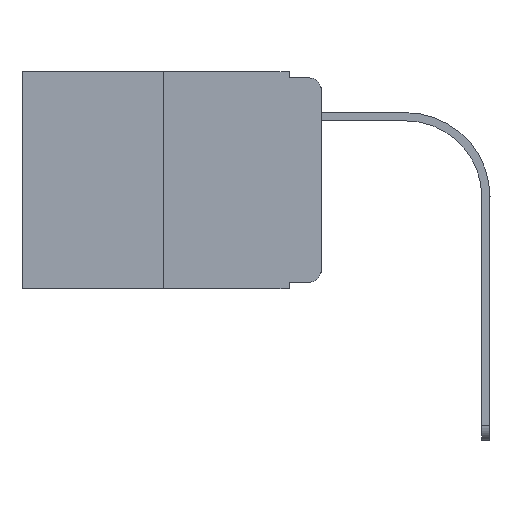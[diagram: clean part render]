
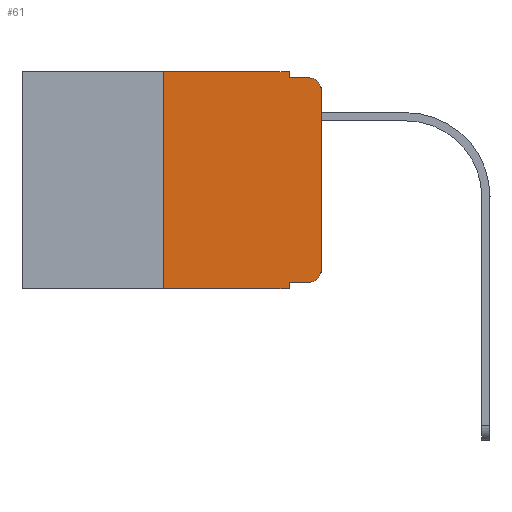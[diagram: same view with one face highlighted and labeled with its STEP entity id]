
A CAD part, left-side view. The second image highlights one B-rep face of the part: STEP entity #61.
In plain terms, the highlighted planar face has unit normal (-1, 0, 0).
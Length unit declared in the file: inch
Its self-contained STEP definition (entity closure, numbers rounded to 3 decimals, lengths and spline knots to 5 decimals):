
#28 = EDGE_CURVE ( 'NONE', #7115, #13252, #396, .T. ) ;
#61 = ADVANCED_FACE ( 'NONE', ( #12761 ), #3958, .F. ) ;
#110 = ORIENTED_EDGE ( 'NONE', *, *, #10447, .T. ) ;
#242 = VECTOR ( 'NONE', #22299, 39.37008 ) ;
#321 = CARTESIAN_POINT ( 'NONE',  ( 0., 0., -0.313 ) ) ;
#396 = LINE ( 'NONE', #7620, #4581 ) ;
#743 = CARTESIAN_POINT ( 'NONE',  ( 0., 0.02, -0.333 ) ) ;
#991 = VERTEX_POINT ( 'NONE', #19166 ) ;
#1076 = CARTESIAN_POINT ( 'NONE',  ( 0., 0.051, -0.333 ) ) ;
#1515 = DIRECTION ( 'NONE',  ( 0., -1., 0. ) ) ;
#1813 = EDGE_CURVE ( 'NONE', #22395, #3302, #22388, .T. ) ;
#1983 = LINE ( 'NONE', #7271, #15126 ) ;
#2420 = ORIENTED_EDGE ( 'NONE', *, *, #20080, .T. ) ;
#2516 = CARTESIAN_POINT ( 'NONE',  ( 0., 0.051, -0.333 ) ) ;
#2645 = CARTESIAN_POINT ( 'NONE',  ( 0., 0.051, 0. ) ) ;
#3045 = VERTEX_POINT ( 'NONE', #3527 ) ;
#3098 = EDGE_CURVE ( 'NONE', #14283, #3302, #21057, .T. ) ;
#3302 = VERTEX_POINT ( 'NONE', #5292 ) ;
#3527 = CARTESIAN_POINT ( 'NONE',  ( 0., 0.25, 0. ) ) ;
#3554 = CARTESIAN_POINT ( 'NONE',  ( 0., 0.25, 0. ) ) ;
#3932 = CIRCLE ( 'NONE', #8331, 0.02 ) ;
#3958 = PLANE ( 'NONE',  #19962 ) ;
#4429 = CARTESIAN_POINT ( 'NONE',  ( 0., 0.02, -0.03 ) ) ;
#4581 = VECTOR ( 'NONE', #19763, 39.37008 ) ;
#4913 = ORIENTED_EDGE ( 'NONE', *, *, #14765, .T. ) ;
#4995 = DIRECTION ( 'NONE',  ( 0., -1., 0. ) ) ;
#5292 = CARTESIAN_POINT ( 'NONE',  ( 0., 0.051, -0.343 ) ) ;
#5351 = CARTESIAN_POINT ( 'NONE',  ( 0., 0.051, 0. ) ) ;
#6211 = ORIENTED_EDGE ( 'NONE', *, *, #28, .F. ) ;
#6414 = AXIS2_PLACEMENT_3D ( 'NONE', #4429, #21852, #18425 ) ;
#6706 = CARTESIAN_POINT ( 'NONE',  ( 0., 0.473, -0.343 ) ) ;
#7115 = VERTEX_POINT ( 'NONE', #2645 ) ;
#7271 = CARTESIAN_POINT ( 'NONE',  ( 0., 0.473, 0. ) ) ;
#7287 = VERTEX_POINT ( 'NONE', #321 ) ;
#7439 = ORIENTED_EDGE ( 'NONE', *, *, #11410, .F. ) ;
#7620 = CARTESIAN_POINT ( 'NONE',  ( 0., 0.051, 0. ) ) ;
#7662 = ORIENTED_EDGE ( 'NONE', *, *, #3098, .F. ) ;
#8331 = AXIS2_PLACEMENT_3D ( 'NONE', #9095, #17698, #16332 ) ;
#8520 = CARTESIAN_POINT ( 'NONE',  ( 0., 0., 0. ) ) ;
#8583 = VERTEX_POINT ( 'NONE', #743 ) ;
#9095 = CARTESIAN_POINT ( 'NONE',  ( 0., 0.02, -0.313 ) ) ;
#9356 = DIRECTION ( 'NONE',  ( 0., 0., 1. ) ) ;
#9366 = VECTOR ( 'NONE', #4995, 39.37008 ) ;
#9940 = CARTESIAN_POINT ( 'NONE',  ( 0., 0.051, -0.01 ) ) ;
#10380 = CARTESIAN_POINT ( 'NONE',  ( 0., 0.051, -0.01 ) ) ;
#10447 = EDGE_CURVE ( 'NONE', #14283, #8583, #17235, .T. ) ;
#10637 = ORIENTED_EDGE ( 'NONE', *, *, #16602, .T. ) ;
#10939 = CARTESIAN_POINT ( 'NONE',  ( 0., 0.473, 0. ) ) ;
#11410 = EDGE_CURVE ( 'NONE', #3045, #7115, #1983, .T. ) ;
#11481 = CARTESIAN_POINT ( 'NONE',  ( 0., 0.25, -0.343 ) ) ;
#12341 = DIRECTION ( 'NONE',  ( 0., 0., -1. ) ) ;
#12761 = FACE_OUTER_BOUND ( 'NONE', #18529, .T. ) ;
#12916 = EDGE_CURVE ( 'NONE', #22395, #3045, #19781, .T. ) ;
#13252 = VERTEX_POINT ( 'NONE', #10380 ) ;
#13697 = VECTOR ( 'NONE', #9356, 39.37008 ) ;
#14283 = VERTEX_POINT ( 'NONE', #2516 ) ;
#14428 = VECTOR ( 'NONE', #21222, 39.37008 ) ;
#14724 = DIRECTION ( 'NONE',  ( 0., 0., -1. ) ) ;
#14765 = EDGE_CURVE ( 'NONE', #15584, #991, #16297, .T. ) ;
#15126 = VECTOR ( 'NONE', #16201, 39.37008 ) ;
#15353 = LINE ( 'NONE', #9940, #242 ) ;
#15584 = VERTEX_POINT ( 'NONE', #20282 ) ;
#16075 = EDGE_CURVE ( 'NONE', #13252, #991, #15353, .T. ) ;
#16201 = DIRECTION ( 'NONE',  ( 0., -1., 0. ) ) ;
#16297 = CIRCLE ( 'NONE', #6414, 0.02 ) ;
#16332 = DIRECTION ( 'NONE',  ( 0., 0., -1. ) ) ;
#16602 = EDGE_CURVE ( 'NONE', #8583, #7287, #3932, .T. ) ;
#17235 = LINE ( 'NONE', #1076, #18387 ) ;
#17516 = VECTOR ( 'NONE', #12341, 39.37008 ) ;
#17698 = DIRECTION ( 'NONE',  ( -1., 0., 0. ) ) ;
#17948 = DIRECTION ( 'NONE',  ( 1., 0., 0. ) ) ;
#18387 = VECTOR ( 'NONE', #1515, 39.37008 ) ;
#18425 = DIRECTION ( 'NONE',  ( 0., 0., -1. ) ) ;
#18529 = EDGE_LOOP ( 'NONE', ( #2420, #4913, #20936, #6211, #7439, #20776, #21105, #7662, #110, #10637 ) ) ;
#19166 = CARTESIAN_POINT ( 'NONE',  ( 0., 0.02, -0.01 ) ) ;
#19763 = DIRECTION ( 'NONE',  ( 0., 0., -1. ) ) ;
#19781 = LINE ( 'NONE', #3554, #13697 ) ;
#19962 = AXIS2_PLACEMENT_3D ( 'NONE', #10939, #17948, #14724 ) ;
#20080 = EDGE_CURVE ( 'NONE', #7287, #15584, #21000, .T. ) ;
#20282 = CARTESIAN_POINT ( 'NONE',  ( 0., 0., -0.03 ) ) ;
#20776 = ORIENTED_EDGE ( 'NONE', *, *, #12916, .F. ) ;
#20936 = ORIENTED_EDGE ( 'NONE', *, *, #16075, .F. ) ;
#21000 = LINE ( 'NONE', #8520, #14428 ) ;
#21057 = LINE ( 'NONE', #5351, #17516 ) ;
#21105 = ORIENTED_EDGE ( 'NONE', *, *, #1813, .T. ) ;
#21222 = DIRECTION ( 'NONE',  ( 0., 0., 1. ) ) ;
#21852 = DIRECTION ( 'NONE',  ( -1., 0., 0. ) ) ;
#22299 = DIRECTION ( 'NONE',  ( 0., -1., 0. ) ) ;
#22388 = LINE ( 'NONE', #6706, #9366 ) ;
#22395 = VERTEX_POINT ( 'NONE', #11481 ) ;
